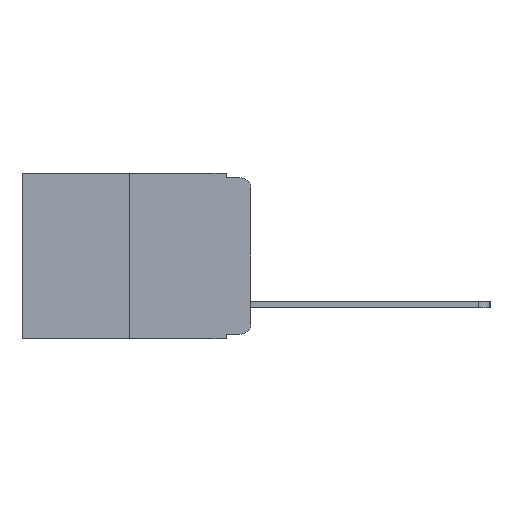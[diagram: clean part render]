
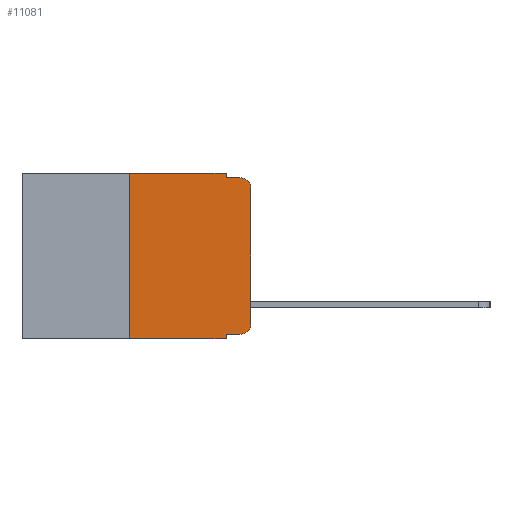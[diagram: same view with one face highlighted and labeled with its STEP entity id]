
A CAD part, left-side view. The second image highlights one B-rep face of the part: STEP entity #11081.
In plain terms, the highlighted planar face has unit normal (-1, 0, 0).
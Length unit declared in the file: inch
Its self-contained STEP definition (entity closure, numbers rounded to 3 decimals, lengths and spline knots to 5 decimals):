
#66 = LINE ( 'NONE', #1217, #2777 ) ;
#89 = ORIENTED_EDGE ( 'NONE', *, *, #418, .F. ) ;
#364 = DIRECTION ( 'NONE',  ( 0., -1., 0. ) ) ;
#418 = EDGE_CURVE ( 'NONE', #6321, #11248, #11374, .T. ) ;
#525 = VECTOR ( 'NONE', #6696, 39.37008 ) ;
#1099 = CARTESIAN_POINT ( 'NONE',  ( 0., 0., -0.313 ) ) ;
#1158 = CARTESIAN_POINT ( 'NONE',  ( 0., 0.02, -0.01 ) ) ;
#1217 = CARTESIAN_POINT ( 'NONE',  ( 0., 0.25, 0. ) ) ;
#1342 = ORIENTED_EDGE ( 'NONE', *, *, #4544, .T. ) ;
#1441 = EDGE_CURVE ( 'NONE', #1575, #6038, #66, .T. ) ;
#1462 = AXIS2_PLACEMENT_3D ( 'NONE', #12924, #9534, #6202 ) ;
#1467 = CARTESIAN_POINT ( 'NONE',  ( 0., 0.051, -0.333 ) ) ;
#1575 = VERTEX_POINT ( 'NONE', #11380 ) ;
#1617 = AXIS2_PLACEMENT_3D ( 'NONE', #2969, #12165, #8738 ) ;
#2150 = CARTESIAN_POINT ( 'NONE',  ( 0., 0.473, 0. ) ) ;
#2342 = VERTEX_POINT ( 'NONE', #1099 ) ;
#2663 = ORIENTED_EDGE ( 'NONE', *, *, #12593, .T. ) ;
#2767 = EDGE_CURVE ( 'NONE', #7898, #5930, #6261, .T. ) ;
#2777 = VECTOR ( 'NONE', #11199, 39.37008 ) ;
#2969 = CARTESIAN_POINT ( 'NONE',  ( 0., 0.02, -0.313 ) ) ;
#3013 = CARTESIAN_POINT ( 'NONE',  ( 0., 0.051, -0.343 ) ) ;
#3134 = EDGE_CURVE ( 'NONE', #7898, #8990, #9787, .T. ) ;
#3279 = ORIENTED_EDGE ( 'NONE', *, *, #4548, .T. ) ;
#3771 = CARTESIAN_POINT ( 'NONE',  ( 0., 0.051, -0.01 ) ) ;
#3834 = EDGE_CURVE ( 'NONE', #11822, #6321, #9204, .T. ) ;
#4133 = CARTESIAN_POINT ( 'NONE',  ( 0., 0.02, -0.03 ) ) ;
#4269 = DIRECTION ( 'NONE',  ( 0., 0., -1. ) ) ;
#4290 = DIRECTION ( 'NONE',  ( -1., 0., 0. ) ) ;
#4291 = VECTOR ( 'NONE', #4317, 39.37008 ) ;
#4317 = DIRECTION ( 'NONE',  ( 0., 0., 1. ) ) ;
#4544 = EDGE_CURVE ( 'NONE', #5933, #11248, #9070, .T. ) ;
#4548 = EDGE_CURVE ( 'NONE', #5930, #2342, #5825, .T. ) ;
#4837 = CARTESIAN_POINT ( 'NONE',  ( 0., 0.051, -0.01 ) ) ;
#5679 = CARTESIAN_POINT ( 'NONE',  ( 0., 0.051, -0.333 ) ) ;
#5825 = CIRCLE ( 'NONE', #1617, 0.02 ) ;
#5901 = VECTOR ( 'NONE', #14420, 39.37008 ) ;
#5930 = VERTEX_POINT ( 'NONE', #11200 ) ;
#5933 = VERTEX_POINT ( 'NONE', #13411 ) ;
#6038 = VERTEX_POINT ( 'NONE', #6661 ) ;
#6202 = DIRECTION ( 'NONE',  ( 0., 0., -1. ) ) ;
#6261 = LINE ( 'NONE', #5679, #13811 ) ;
#6321 = VERTEX_POINT ( 'NONE', #4837 ) ;
#6654 = ORIENTED_EDGE ( 'NONE', *, *, #3134, .F. ) ;
#6661 = CARTESIAN_POINT ( 'NONE',  ( 0., 0.25, 0. ) ) ;
#6696 = DIRECTION ( 'NONE',  ( 0., -1., 0. ) ) ;
#6891 = ORIENTED_EDGE ( 'NONE', *, *, #2767, .T. ) ;
#6981 = LINE ( 'NONE', #13707, #525 ) ;
#7898 = VERTEX_POINT ( 'NONE', #1467 ) ;
#8040 = DIRECTION ( 'NONE',  ( 0., 0., -1. ) ) ;
#8152 = CARTESIAN_POINT ( 'NONE',  ( 0., 0.051, 0. ) ) ;
#8467 = PLANE ( 'NONE',  #1462 ) ;
#8718 = CARTESIAN_POINT ( 'NONE',  ( 0., 0.051, 0. ) ) ;
#8738 = DIRECTION ( 'NONE',  ( 0., 0., -1. ) ) ;
#8864 = VECTOR ( 'NONE', #4269, 39.37008 ) ;
#8990 = VERTEX_POINT ( 'NONE', #3013 ) ;
#9070 = CIRCLE ( 'NONE', #11857, 0.02 ) ;
#9204 = LINE ( 'NONE', #10292, #13663 ) ;
#9249 = EDGE_CURVE ( 'NONE', #6038, #11822, #12132, .T. ) ;
#9534 = DIRECTION ( 'NONE',  ( 1., 0., 0. ) ) ;
#9732 = DIRECTION ( 'NONE',  ( 0., 0., -1. ) ) ;
#9787 = LINE ( 'NONE', #8718, #8864 ) ;
#9844 = LINE ( 'NONE', #9981, #4291 ) ;
#9981 = CARTESIAN_POINT ( 'NONE',  ( 0., 0., 0. ) ) ;
#10292 = CARTESIAN_POINT ( 'NONE',  ( 0., 0.051, 0. ) ) ;
#10652 = ORIENTED_EDGE ( 'NONE', *, *, #3834, .F. ) ;
#11081 = ADVANCED_FACE ( 'NONE', ( #12990 ), #8467, .F. ) ;
#11199 = DIRECTION ( 'NONE',  ( 0., 0., 1. ) ) ;
#11200 = CARTESIAN_POINT ( 'NONE',  ( 0., 0.02, -0.333 ) ) ;
#11248 = VERTEX_POINT ( 'NONE', #1158 ) ;
#11374 = LINE ( 'NONE', #3771, #12848 ) ;
#11380 = CARTESIAN_POINT ( 'NONE',  ( 0., 0.25, -0.343 ) ) ;
#11822 = VERTEX_POINT ( 'NONE', #8152 ) ;
#11857 = AXIS2_PLACEMENT_3D ( 'NONE', #4133, #4290, #9732 ) ;
#11858 = EDGE_CURVE ( 'NONE', #1575, #8990, #6981, .T. ) ;
#11985 = ORIENTED_EDGE ( 'NONE', *, *, #9249, .F. ) ;
#12002 = ORIENTED_EDGE ( 'NONE', *, *, #1441, .F. ) ;
#12051 = ORIENTED_EDGE ( 'NONE', *, *, #11858, .T. ) ;
#12132 = LINE ( 'NONE', #2150, #5901 ) ;
#12165 = DIRECTION ( 'NONE',  ( -1., 0., 0. ) ) ;
#12593 = EDGE_CURVE ( 'NONE', #2342, #5933, #9844, .T. ) ;
#12848 = VECTOR ( 'NONE', #364, 39.37008 ) ;
#12924 = CARTESIAN_POINT ( 'NONE',  ( 0., 0.473, 0. ) ) ;
#12990 = FACE_OUTER_BOUND ( 'NONE', #13567, .T. ) ;
#13411 = CARTESIAN_POINT ( 'NONE',  ( 0., 0., -0.03 ) ) ;
#13478 = DIRECTION ( 'NONE',  ( 0., -1., 0. ) ) ;
#13567 = EDGE_LOOP ( 'NONE', ( #2663, #1342, #89, #10652, #11985, #12002, #12051, #6654, #6891, #3279 ) ) ;
#13663 = VECTOR ( 'NONE', #8040, 39.37008 ) ;
#13707 = CARTESIAN_POINT ( 'NONE',  ( 0., 0.473, -0.343 ) ) ;
#13811 = VECTOR ( 'NONE', #13478, 39.37008 ) ;
#14420 = DIRECTION ( 'NONE',  ( 0., -1., 0. ) ) ;
